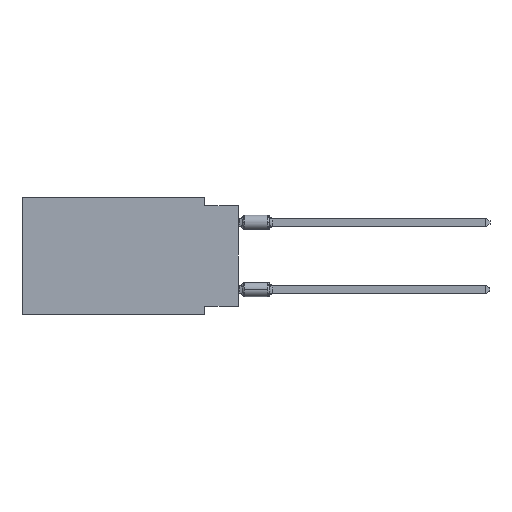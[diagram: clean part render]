
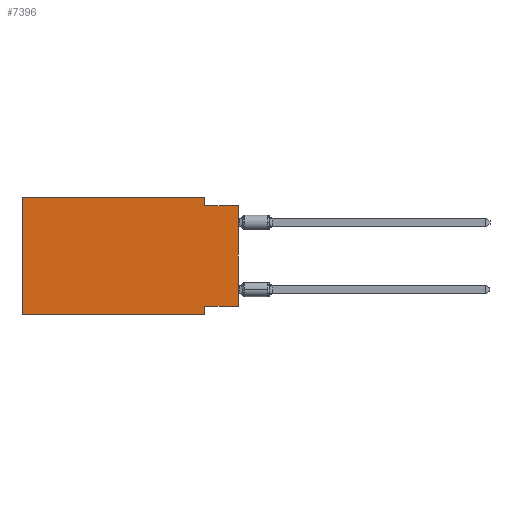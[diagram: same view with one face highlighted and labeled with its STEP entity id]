
A CAD part, left-side view. The second image highlights one B-rep face of the part: STEP entity #7396.
In plain terms, the highlighted planar face has unit normal (-1, 0, 0).
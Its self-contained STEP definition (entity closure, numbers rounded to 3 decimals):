
#92 = CARTESIAN_POINT ( 'NONE',  ( 0., 16.383, -8.89 ) ) ;
#94 = ORIENTED_EDGE ( 'NONE', *, *, #8799, .F. ) ;
#171 = LINE ( 'NONE', #6033, #15068 ) ;
#450 = EDGE_CURVE ( 'NONE', #6075, #10808, #13076, .T. ) ;
#472 = DIRECTION ( 'NONE',  ( 0., 0., 1. ) ) ;
#532 = EDGE_CURVE ( 'NONE', #5071, #5521, #938, .T. ) ;
#543 = DIRECTION ( 'NONE',  ( 1., 0., 0. ) ) ;
#808 = DIRECTION ( 'NONE',  ( 0., 0., -1. ) ) ;
#938 = LINE ( 'NONE', #4256, #11814 ) ;
#1163 = VERTEX_POINT ( 'NONE', #10606 ) ;
#1440 = CARTESIAN_POINT ( 'NONE',  ( 0., 0., -8.255 ) ) ;
#1705 = CARTESIAN_POINT ( 'NONE',  ( 0., 16.383, 0. ) ) ;
#1810 = LINE ( 'NONE', #2746, #11602 ) ;
#2040 = VECTOR ( 'NONE', #5602, 1000. ) ;
#2199 = CARTESIAN_POINT ( 'NONE',  ( 0., 2.54, 0. ) ) ;
#2674 = LINE ( 'NONE', #1440, #6337 ) ;
#2746 = CARTESIAN_POINT ( 'NONE',  ( 0., 16.383, 0. ) ) ;
#2867 = EDGE_CURVE ( 'NONE', #10165, #4045, #3360, .T. ) ;
#3286 = CARTESIAN_POINT ( 'NONE',  ( 0., 16.383, -8.89 ) ) ;
#3360 = LINE ( 'NONE', #2199, #14453 ) ;
#3984 = DIRECTION ( 'NONE',  ( 0., 1., 0. ) ) ;
#4045 = VERTEX_POINT ( 'NONE', #11062 ) ;
#4256 = CARTESIAN_POINT ( 'NONE',  ( 0., 2.54, -8.89 ) ) ;
#4642 = VECTOR ( 'NONE', #13004, 1000. ) ;
#4718 = ORIENTED_EDGE ( 'NONE', *, *, #7177, .F. ) ;
#5003 = ORIENTED_EDGE ( 'NONE', *, *, #10110, .F. ) ;
#5045 = CARTESIAN_POINT ( 'NONE',  ( 0., 2.54, -8.89 ) ) ;
#5071 = VERTEX_POINT ( 'NONE', #5208 ) ;
#5208 = CARTESIAN_POINT ( 'NONE',  ( 0., 2.54, -8.255 ) ) ;
#5488 = DIRECTION ( 'NONE',  ( 0., 0., -1. ) ) ;
#5521 = VERTEX_POINT ( 'NONE', #5045 ) ;
#5602 = DIRECTION ( 'NONE',  ( 0., -1., 0. ) ) ;
#5899 = ORIENTED_EDGE ( 'NONE', *, *, #532, .F. ) ;
#6033 = CARTESIAN_POINT ( 'NONE',  ( 0., 16.383, 0. ) ) ;
#6035 = LINE ( 'NONE', #92, #12112 ) ;
#6075 = VERTEX_POINT ( 'NONE', #6467 ) ;
#6337 = VECTOR ( 'NONE', #3984, 1000. ) ;
#6467 = CARTESIAN_POINT ( 'NONE',  ( 0., 0., -8.255 ) ) ;
#6961 = ORIENTED_EDGE ( 'NONE', *, *, #2867, .F. ) ;
#7177 = EDGE_CURVE ( 'NONE', #8470, #1163, #171, .T. ) ;
#7396 = ADVANCED_FACE ( 'NONE', ( #12255 ), #13541, .F. ) ;
#8279 = ORIENTED_EDGE ( 'NONE', *, *, #13295, .F. ) ;
#8470 = VERTEX_POINT ( 'NONE', #3286 ) ;
#8620 = ORIENTED_EDGE ( 'NONE', *, *, #450, .T. ) ;
#8799 = EDGE_CURVE ( 'NONE', #6075, #5071, #2674, .T. ) ;
#9008 = DIRECTION ( 'NONE',  ( 0., 0., -1. ) ) ;
#9935 = AXIS2_PLACEMENT_3D ( 'NONE', #1705, #543, #9008 ) ;
#10110 = EDGE_CURVE ( 'NONE', #1163, #10165, #1810, .T. ) ;
#10165 = VERTEX_POINT ( 'NONE', #10272 ) ;
#10272 = CARTESIAN_POINT ( 'NONE',  ( 0., 2.54, 0. ) ) ;
#10606 = CARTESIAN_POINT ( 'NONE',  ( 0., 16.383, 0. ) ) ;
#10614 = CARTESIAN_POINT ( 'NONE',  ( 0., 0., 0. ) ) ;
#10664 = EDGE_CURVE ( 'NONE', #8470, #5521, #6035, .T. ) ;
#10808 = VERTEX_POINT ( 'NONE', #14170 ) ;
#10977 = DIRECTION ( 'NONE',  ( 0., -1., 0. ) ) ;
#11062 = CARTESIAN_POINT ( 'NONE',  ( 0., 2.54, -0.635 ) ) ;
#11602 = VECTOR ( 'NONE', #10977, 1000. ) ;
#11814 = VECTOR ( 'NONE', #5488, 1000. ) ;
#11861 = DIRECTION ( 'NONE',  ( 0., -1., 0. ) ) ;
#12112 = VECTOR ( 'NONE', #11861, 1000. ) ;
#12255 = FACE_OUTER_BOUND ( 'NONE', #12850, .T. ) ;
#12454 = ORIENTED_EDGE ( 'NONE', *, *, #10664, .T. ) ;
#12850 = EDGE_LOOP ( 'NONE', ( #8620, #8279, #6961, #5003, #4718, #12454, #5899, #94 ) ) ;
#13004 = DIRECTION ( 'NONE',  ( 0., 0., 1. ) ) ;
#13076 = LINE ( 'NONE', #10614, #4642 ) ;
#13295 = EDGE_CURVE ( 'NONE', #4045, #10808, #14894, .T. ) ;
#13541 = PLANE ( 'NONE',  #9935 ) ;
#14170 = CARTESIAN_POINT ( 'NONE',  ( 0., 0., -0.635 ) ) ;
#14453 = VECTOR ( 'NONE', #808, 1000. ) ;
#14813 = CARTESIAN_POINT ( 'NONE',  ( 0., 0., -0.635 ) ) ;
#14894 = LINE ( 'NONE', #14813, #2040 ) ;
#15068 = VECTOR ( 'NONE', #472, 1000. ) ;
